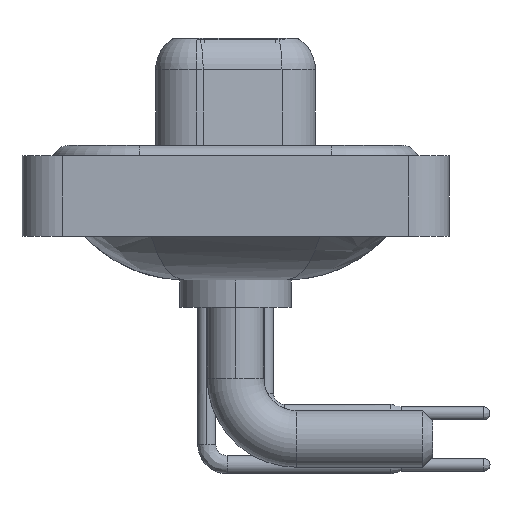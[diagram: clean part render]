
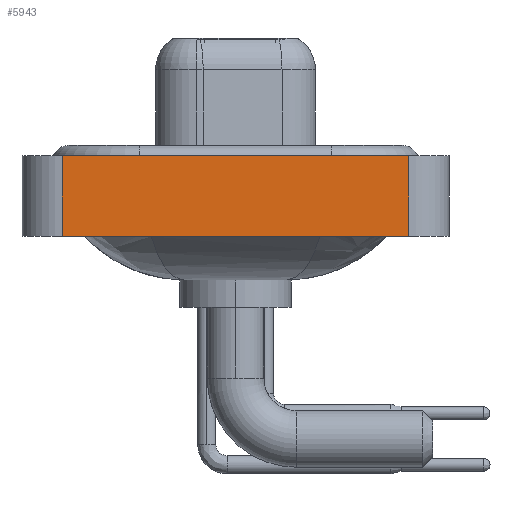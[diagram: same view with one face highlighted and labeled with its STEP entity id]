
A CAD part, left-side view. The second image highlights one B-rep face of the part: STEP entity #5943.
In plain terms, the highlighted planar face has unit normal (-1, 0, 0).
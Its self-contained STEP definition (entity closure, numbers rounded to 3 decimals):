
#190 = ORIENTED_EDGE ( 'NONE', *, *, #11651, .T. ) ;
#1265 = DIRECTION ( 'NONE',  ( 0., -1., 0. ) ) ;
#1829 = LINE ( 'NONE', #15502, #7437 ) ;
#3224 = VECTOR ( 'NONE', #19255, 1000. ) ;
#3853 = PLANE ( 'NONE',  #12033 ) ;
#4252 = VERTEX_POINT ( 'NONE', #9390 ) ;
#5030 = LINE ( 'NONE', #8986, #20299 ) ;
#5192 = ORIENTED_EDGE ( 'NONE', *, *, #7298, .F. ) ;
#5943 = ADVANCED_FACE ( 'NONE', ( #15166 ), #3853, .T. ) ;
#6834 = VERTEX_POINT ( 'NONE', #19839 ) ;
#7298 = EDGE_CURVE ( 'NONE', #22208, #6834, #15524, .T. ) ;
#7437 = VECTOR ( 'NONE', #15382, 1000. ) ;
#7917 = CARTESIAN_POINT ( 'NONE',  ( -7.35, -8.55, -3.6 ) ) ;
#8263 = VECTOR ( 'NONE', #1265, 1000. ) ;
#8986 = CARTESIAN_POINT ( 'NONE',  ( -7.35, 8.55, -3.6 ) ) ;
#9390 = CARTESIAN_POINT ( 'NONE',  ( -7.35, 8.55, -3.6 ) ) ;
#11651 = EDGE_CURVE ( 'NONE', #11660, #6834, #1829, .T. ) ;
#11660 = VERTEX_POINT ( 'NONE', #7917 ) ;
#12033 = AXIS2_PLACEMENT_3D ( 'NONE', #19298, #20875, #22988 ) ;
#13689 = EDGE_CURVE ( 'NONE', #4252, #22208, #5030, .T. ) ;
#14265 = CARTESIAN_POINT ( 'NONE',  ( -7.35, 8.55, 0.4 ) ) ;
#14278 = EDGE_LOOP ( 'NONE', ( #190, #5192, #14633, #23259 ) ) ;
#14633 = ORIENTED_EDGE ( 'NONE', *, *, #13689, .F. ) ;
#15166 = FACE_OUTER_BOUND ( 'NONE', #14278, .T. ) ;
#15382 = DIRECTION ( 'NONE',  ( 0., 0., 1. ) ) ;
#15502 = CARTESIAN_POINT ( 'NONE',  ( -7.35, -8.55, -3.6 ) ) ;
#15524 = LINE ( 'NONE', #20998, #3224 ) ;
#18327 = LINE ( 'NONE', #24031, #8263 ) ;
#18566 = DIRECTION ( 'NONE',  ( 0., 0., 1. ) ) ;
#19255 = DIRECTION ( 'NONE',  ( 0., -1., 0. ) ) ;
#19298 = CARTESIAN_POINT ( 'NONE',  ( -7.35, -8.55, -3.6 ) ) ;
#19670 = EDGE_CURVE ( 'NONE', #4252, #11660, #18327, .T. ) ;
#19839 = CARTESIAN_POINT ( 'NONE',  ( -7.35, -8.55, 0.4 ) ) ;
#20299 = VECTOR ( 'NONE', #18566, 1000. ) ;
#20875 = DIRECTION ( 'NONE',  ( -1., 0., 0. ) ) ;
#20998 = CARTESIAN_POINT ( 'NONE',  ( -7.35, -8.55, 0.4 ) ) ;
#22208 = VERTEX_POINT ( 'NONE', #14265 ) ;
#22988 = DIRECTION ( 'NONE',  ( 0., 0., 1. ) ) ;
#23259 = ORIENTED_EDGE ( 'NONE', *, *, #19670, .T. ) ;
#24031 = CARTESIAN_POINT ( 'NONE',  ( -7.35, -8.55, -3.6 ) ) ;
